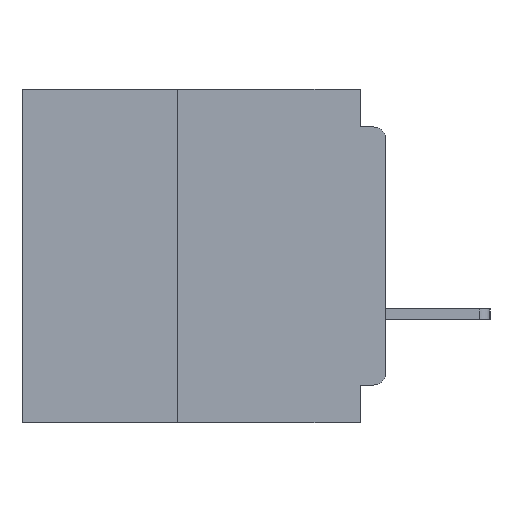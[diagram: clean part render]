
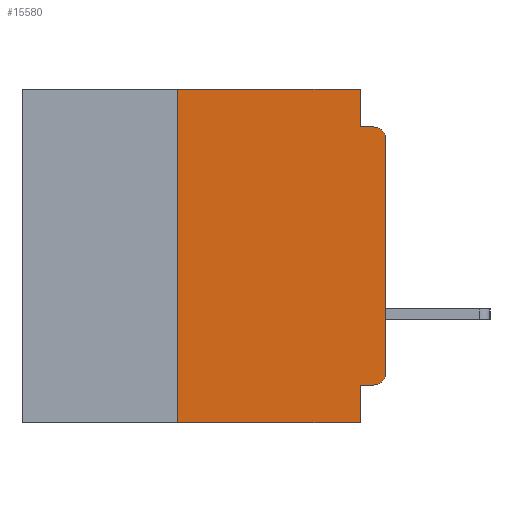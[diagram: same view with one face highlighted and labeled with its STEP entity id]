
A CAD part, left-side view. The second image highlights one B-rep face of the part: STEP entity #15580.
In plain terms, the highlighted planar face has unit normal (-1, 0, 0).
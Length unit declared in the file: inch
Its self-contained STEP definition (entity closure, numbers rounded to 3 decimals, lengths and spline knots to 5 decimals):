
#554 = VERTEX_POINT ( 'NONE', #21670 ) ;
#2032 = VERTEX_POINT ( 'NONE', #22584 ) ;
#2491 = CARTESIAN_POINT ( 'NONE',  ( 0., 0., 0. ) ) ;
#5332 = CARTESIAN_POINT ( 'NONE',  ( 0., 0.015, -0.045 ) ) ;
#5885 = CARTESIAN_POINT ( 'NONE',  ( 0., 0.437, 0. ) ) ;
#6512 = VERTEX_POINT ( 'NONE', #25124 ) ;
#8499 = CIRCLE ( 'NONE', #43476, 0.015 ) ;
#9462 = VECTOR ( 'NONE', #29158, 39.37008 ) ;
#9896 = CARTESIAN_POINT ( 'NONE',  ( 0., 0.25, -0.4 ) ) ;
#11704 = DIRECTION ( 'NONE',  ( 0., 0., -1. ) ) ;
#12767 = ORIENTED_EDGE ( 'NONE', *, *, #40601, .F. ) ;
#12920 = CARTESIAN_POINT ( 'NONE',  ( 0., 0.015, -0.34 ) ) ;
#13329 = EDGE_LOOP ( 'NONE', ( #63529, #50715, #47136, #49933, #43809, #37409, #47183, #40660, #12767, #47662 ) ) ;
#13498 = CARTESIAN_POINT ( 'NONE',  ( 0., 0., -0.355 ) ) ;
#14035 = CARTESIAN_POINT ( 'NONE',  ( 0., 0., -0.045 ) ) ;
#14845 = DIRECTION ( 'NONE',  ( 0., 0., -1. ) ) ;
#15580 = ADVANCED_FACE ( 'NONE', ( #49375 ), #16108, .F. ) ;
#16108 = PLANE ( 'NONE',  #20459 ) ;
#16224 = VERTEX_POINT ( 'NONE', #16251 ) ;
#16251 = CARTESIAN_POINT ( 'NONE',  ( 0., 0.015, -0.355 ) ) ;
#16830 = CIRCLE ( 'NONE', #34133, 0.015 ) ;
#17973 = DIRECTION ( 'NONE',  ( 0., 0., -1. ) ) ;
#19870 = LINE ( 'NONE', #13498, #48234 ) ;
#19910 = LINE ( 'NONE', #9896, #46675 ) ;
#20459 = AXIS2_PLACEMENT_3D ( 'NONE', #51349, #61496, #31269 ) ;
#21299 = EDGE_CURVE ( 'NONE', #6512, #60435, #22810, .T. ) ;
#21405 = LINE ( 'NONE', #50092, #33204 ) ;
#21670 = CARTESIAN_POINT ( 'NONE',  ( 0., 0.25, 0. ) ) ;
#22584 = CARTESIAN_POINT ( 'NONE',  ( 0., 0.031, 0. ) ) ;
#22699 = VERTEX_POINT ( 'NONE', #50748 ) ;
#22810 = LINE ( 'NONE', #14035, #9462 ) ;
#25124 = CARTESIAN_POINT ( 'NONE',  ( 0., 0.031, -0.045 ) ) ;
#26051 = VECTOR ( 'NONE', #52915, 39.37008 ) ;
#29158 = DIRECTION ( 'NONE',  ( 0., -1., 0. ) ) ;
#29277 = CARTESIAN_POINT ( 'NONE',  ( 0., 0.015, -0.06 ) ) ;
#29740 = EDGE_CURVE ( 'NONE', #47415, #58488, #52933, .T. ) ;
#31269 = DIRECTION ( 'NONE',  ( 0., 0., -1. ) ) ;
#31280 = CARTESIAN_POINT ( 'NONE',  ( 0., 0.437, -0.4 ) ) ;
#33204 = VECTOR ( 'NONE', #14845, 39.37008 ) ;
#33590 = LINE ( 'NONE', #62138, #58894 ) ;
#33737 = EDGE_CURVE ( 'NONE', #22699, #48744, #39390, .T. ) ;
#34133 = AXIS2_PLACEMENT_3D ( 'NONE', #12920, #48116, #17973 ) ;
#34352 = DIRECTION ( 'NONE',  ( 0., 0., -1. ) ) ;
#37075 = CARTESIAN_POINT ( 'NONE',  ( 0., 0.031, -0.355 ) ) ;
#37409 = ORIENTED_EDGE ( 'NONE', *, *, #64648, .F. ) ;
#39166 = EDGE_CURVE ( 'NONE', #16224, #22699, #16830, .T. ) ;
#39390 = LINE ( 'NONE', #2491, #26051 ) ;
#39974 = DIRECTION ( 'NONE',  ( 0., 0., 1. ) ) ;
#40601 = EDGE_CURVE ( 'NONE', #16224, #41638, #19870, .T. ) ;
#40660 = ORIENTED_EDGE ( 'NONE', *, *, #62530, .F. ) ;
#41336 = CARTESIAN_POINT ( 'NONE',  ( 0., 0., -0.06 ) ) ;
#41638 = VERTEX_POINT ( 'NONE', #37075 ) ;
#41658 = CARTESIAN_POINT ( 'NONE',  ( 0., 0.031, -0.4 ) ) ;
#42440 = EDGE_CURVE ( 'NONE', #2032, #6512, #21405, .T. ) ;
#43476 = AXIS2_PLACEMENT_3D ( 'NONE', #29277, #64596, #34352 ) ;
#43623 = DIRECTION ( 'NONE',  ( 0., 1., 0. ) ) ;
#43809 = ORIENTED_EDGE ( 'NONE', *, *, #55807, .F. ) ;
#44254 = VECTOR ( 'NONE', #61356, 39.37008 ) ;
#45821 = LINE ( 'NONE', #5885, #44254 ) ;
#46675 = VECTOR ( 'NONE', #39974, 39.37008 ) ;
#47136 = ORIENTED_EDGE ( 'NONE', *, *, #21299, .F. ) ;
#47183 = ORIENTED_EDGE ( 'NONE', *, *, #29740, .T. ) ;
#47415 = VERTEX_POINT ( 'NONE', #59045 ) ;
#47662 = ORIENTED_EDGE ( 'NONE', *, *, #39166, .T. ) ;
#48116 = DIRECTION ( 'NONE',  ( -1., 0., 0. ) ) ;
#48234 = VECTOR ( 'NONE', #43623, 39.37008 ) ;
#48744 = VERTEX_POINT ( 'NONE', #41336 ) ;
#49375 = FACE_OUTER_BOUND ( 'NONE', #13329, .T. ) ;
#49933 = ORIENTED_EDGE ( 'NONE', *, *, #42440, .F. ) ;
#50092 = CARTESIAN_POINT ( 'NONE',  ( 0., 0.031, 0. ) ) ;
#50715 = ORIENTED_EDGE ( 'NONE', *, *, #62130, .T. ) ;
#50748 = CARTESIAN_POINT ( 'NONE',  ( 0., 0., -0.34 ) ) ;
#51349 = CARTESIAN_POINT ( 'NONE',  ( 0., 0.437, 0. ) ) ;
#52915 = DIRECTION ( 'NONE',  ( 0., 0., 1. ) ) ;
#52933 = LINE ( 'NONE', #31280, #61592 ) ;
#55807 = EDGE_CURVE ( 'NONE', #554, #2032, #45821, .T. ) ;
#58488 = VERTEX_POINT ( 'NONE', #41658 ) ;
#58894 = VECTOR ( 'NONE', #11704, 39.37008 ) ;
#59045 = CARTESIAN_POINT ( 'NONE',  ( 0., 0.25, -0.4 ) ) ;
#60435 = VERTEX_POINT ( 'NONE', #5332 ) ;
#61356 = DIRECTION ( 'NONE',  ( 0., -1., 0. ) ) ;
#61496 = DIRECTION ( 'NONE',  ( 1., 0., 0. ) ) ;
#61592 = VECTOR ( 'NONE', #61717, 39.37008 ) ;
#61717 = DIRECTION ( 'NONE',  ( 0., -1., 0. ) ) ;
#62130 = EDGE_CURVE ( 'NONE', #48744, #60435, #8499, .T. ) ;
#62138 = CARTESIAN_POINT ( 'NONE',  ( 0., 0.031, -0.4 ) ) ;
#62530 = EDGE_CURVE ( 'NONE', #41638, #58488, #33590, .T. ) ;
#63529 = ORIENTED_EDGE ( 'NONE', *, *, #33737, .T. ) ;
#64596 = DIRECTION ( 'NONE',  ( -1., 0., 0. ) ) ;
#64648 = EDGE_CURVE ( 'NONE', #47415, #554, #19910, .T. ) ;
